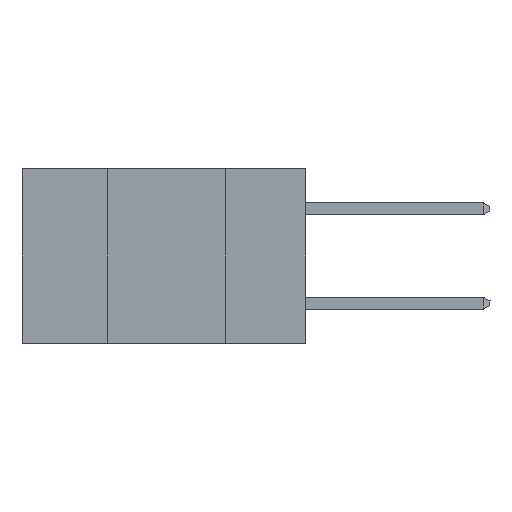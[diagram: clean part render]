
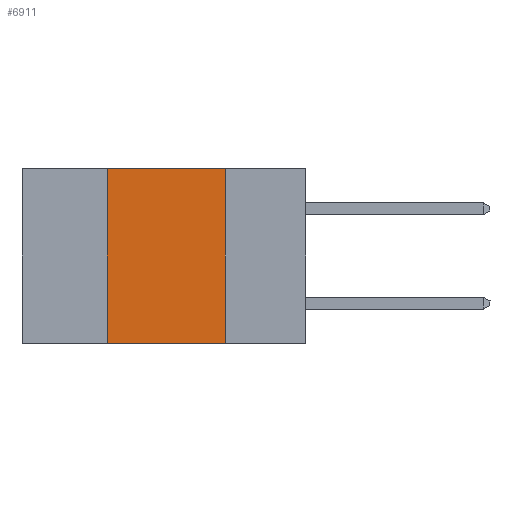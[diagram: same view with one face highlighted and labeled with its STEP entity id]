
A CAD part, left-side view. The second image highlights one B-rep face of the part: STEP entity #6911.
In plain terms, the highlighted planar face has unit normal (-1, 0, 0).
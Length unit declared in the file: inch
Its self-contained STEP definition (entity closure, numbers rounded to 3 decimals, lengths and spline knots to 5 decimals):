
#141 = CARTESIAN_POINT ( 'NONE',  ( 0., 0.42, -0.37 ) ) ;
#699 = CARTESIAN_POINT ( 'NONE',  ( 0., 0.42, 0. ) ) ;
#758 = ORIENTED_EDGE ( 'NONE', *, *, #15102, .F. ) ;
#1732 = PLANE ( 'NONE',  #2974 ) ;
#2028 = CARTESIAN_POINT ( 'NONE',  ( 0., 0.6, 0. ) ) ;
#2217 = VECTOR ( 'NONE', #17175, 39.37008 ) ;
#2243 = VECTOR ( 'NONE', #10662, 39.37008 ) ;
#2700 = ORIENTED_EDGE ( 'NONE', *, *, #13861, .F. ) ;
#2974 = AXIS2_PLACEMENT_3D ( 'NONE', #2028, #11692, #17301 ) ;
#3272 = VECTOR ( 'NONE', #13148, 39.37008 ) ;
#3482 = CARTESIAN_POINT ( 'NONE',  ( 0., 0.6, -0.37 ) ) ;
#3895 = CARTESIAN_POINT ( 'NONE',  ( 0., 0.17, 0. ) ) ;
#4367 = LINE ( 'NONE', #3482, #2217 ) ;
#4924 = VERTEX_POINT ( 'NONE', #141 ) ;
#6667 = LINE ( 'NONE', #7657, #3272 ) ;
#6911 = ADVANCED_FACE ( 'NONE', ( #10736 ), #1732, .F. ) ;
#6938 = VERTEX_POINT ( 'NONE', #16327 ) ;
#7657 = CARTESIAN_POINT ( 'NONE',  ( 0., 0.6, 0. ) ) ;
#8565 = VERTEX_POINT ( 'NONE', #10543 ) ;
#8941 = LINE ( 'NONE', #699, #16235 ) ;
#9412 = ORIENTED_EDGE ( 'NONE', *, *, #14060, .F. ) ;
#10300 = DIRECTION ( 'NONE',  ( 0., 0., 1. ) ) ;
#10543 = CARTESIAN_POINT ( 'NONE',  ( 0., 0.17, 0. ) ) ;
#10662 = DIRECTION ( 'NONE',  ( 0., 0., -1. ) ) ;
#10736 = FACE_OUTER_BOUND ( 'NONE', #11153, .T. ) ;
#11153 = EDGE_LOOP ( 'NONE', ( #9412, #758, #2700, #15439 ) ) ;
#11692 = DIRECTION ( 'NONE',  ( 1., 0., 0. ) ) ;
#13148 = DIRECTION ( 'NONE',  ( 0., -1., 0. ) ) ;
#13861 = EDGE_CURVE ( 'NONE', #4924, #17726, #8941, .T. ) ;
#14060 = EDGE_CURVE ( 'NONE', #8565, #6938, #14295, .T. ) ;
#14295 = LINE ( 'NONE', #3895, #2243 ) ;
#14630 = EDGE_CURVE ( 'NONE', #4924, #6938, #4367, .T. ) ;
#14782 = CARTESIAN_POINT ( 'NONE',  ( 0., 0.42, 0. ) ) ;
#15102 = EDGE_CURVE ( 'NONE', #17726, #8565, #6667, .T. ) ;
#15439 = ORIENTED_EDGE ( 'NONE', *, *, #14630, .T. ) ;
#16235 = VECTOR ( 'NONE', #10300, 39.37008 ) ;
#16327 = CARTESIAN_POINT ( 'NONE',  ( 0., 0.17, -0.37 ) ) ;
#17175 = DIRECTION ( 'NONE',  ( 0., -1., 0. ) ) ;
#17301 = DIRECTION ( 'NONE',  ( 0., 0., -1. ) ) ;
#17726 = VERTEX_POINT ( 'NONE', #14782 ) ;
